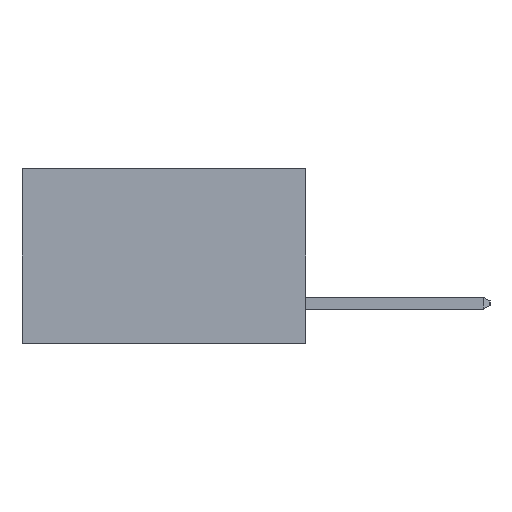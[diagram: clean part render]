
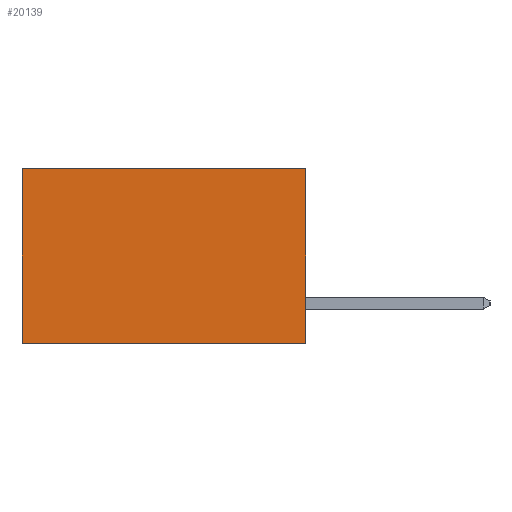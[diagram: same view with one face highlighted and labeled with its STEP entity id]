
A CAD part, left-side view. The second image highlights one B-rep face of the part: STEP entity #20139.
In plain terms, the highlighted planar face has unit normal (-1, 0, 0).
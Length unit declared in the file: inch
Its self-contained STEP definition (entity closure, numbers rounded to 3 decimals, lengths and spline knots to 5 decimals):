
#168 = CARTESIAN_POINT ( 'NONE',  ( 0.298, 0., 0. ) ) ;
#209 = EDGE_CURVE ( 'NONE', #4600, #1211, #21123, .T. ) ;
#226 = CARTESIAN_POINT ( 'NONE',  ( 0.298, 0.6, 0. ) ) ;
#1211 = VERTEX_POINT ( 'NONE', #16521 ) ;
#2037 = DIRECTION ( 'NONE',  ( 0., 0., -1. ) ) ;
#2261 = ORIENTED_EDGE ( 'NONE', *, *, #14729, .F. ) ;
#2875 = LINE ( 'NONE', #6294, #11729 ) ;
#3314 = PLANE ( 'NONE',  #3392 ) ;
#3392 = AXIS2_PLACEMENT_3D ( 'NONE', #15649, #5333, #17347 ) ;
#3395 = VECTOR ( 'NONE', #12842, 39.37008 ) ;
#4600 = VERTEX_POINT ( 'NONE', #168 ) ;
#5333 = DIRECTION ( 'NONE',  ( 1., 0., 0. ) ) ;
#6015 = VERTEX_POINT ( 'NONE', #12880 ) ;
#6294 = CARTESIAN_POINT ( 'NONE',  ( 0.298, 0., -0.37 ) ) ;
#7123 = LINE ( 'NONE', #226, #11198 ) ;
#8524 = CARTESIAN_POINT ( 'NONE',  ( 0.298, 0., 0. ) ) ;
#10765 = ORIENTED_EDGE ( 'NONE', *, *, #20019, .T. ) ;
#11198 = VECTOR ( 'NONE', #2037, 39.37008 ) ;
#11729 = VECTOR ( 'NONE', #14866, 39.37008 ) ;
#12842 = DIRECTION ( 'NONE',  ( 0., 0., -1. ) ) ;
#12880 = CARTESIAN_POINT ( 'NONE',  ( 0.298, 0.6, 0. ) ) ;
#14729 = EDGE_CURVE ( 'NONE', #1211, #16251, #2875, .T. ) ;
#14866 = DIRECTION ( 'NONE',  ( 0., 1., 0. ) ) ;
#15134 = EDGE_CURVE ( 'NONE', #6015, #16251, #7123, .T. ) ;
#15633 = ORIENTED_EDGE ( 'NONE', *, *, #209, .F. ) ;
#15649 = CARTESIAN_POINT ( 'NONE',  ( 0.298, 0., 0. ) ) ;
#16251 = VERTEX_POINT ( 'NONE', #22001 ) ;
#16314 = VECTOR ( 'NONE', #18650, 39.37008 ) ;
#16521 = CARTESIAN_POINT ( 'NONE',  ( 0.298, 0., -0.37 ) ) ;
#16720 = CARTESIAN_POINT ( 'NONE',  ( 0.298, 0., 0. ) ) ;
#17347 = DIRECTION ( 'NONE',  ( 0., 0., -1. ) ) ;
#18129 = FACE_OUTER_BOUND ( 'NONE', #21862, .T. ) ;
#18650 = DIRECTION ( 'NONE',  ( 0., 1., 0. ) ) ;
#20019 = EDGE_CURVE ( 'NONE', #4600, #6015, #21224, .T. ) ;
#20139 = ADVANCED_FACE ( 'NONE', ( #18129 ), #3314, .F. ) ;
#21123 = LINE ( 'NONE', #16720, #3395 ) ;
#21224 = LINE ( 'NONE', #8524, #16314 ) ;
#21843 = ORIENTED_EDGE ( 'NONE', *, *, #15134, .T. ) ;
#21862 = EDGE_LOOP ( 'NONE', ( #21843, #2261, #15633, #10765 ) ) ;
#22001 = CARTESIAN_POINT ( 'NONE',  ( 0.298, 0.6, -0.37 ) ) ;
